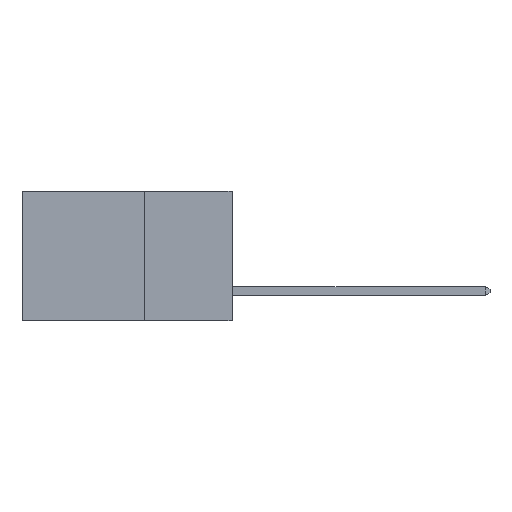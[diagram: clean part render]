
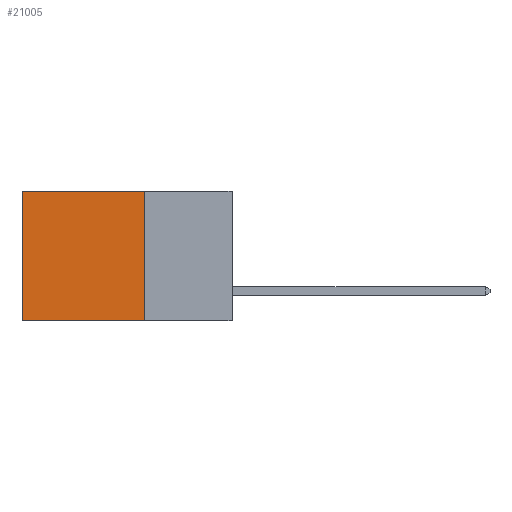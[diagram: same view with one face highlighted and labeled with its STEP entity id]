
A CAD part, left-side view. The second image highlights one B-rep face of the part: STEP entity #21005.
In plain terms, the highlighted planar face has unit normal (-1, 0, 0).
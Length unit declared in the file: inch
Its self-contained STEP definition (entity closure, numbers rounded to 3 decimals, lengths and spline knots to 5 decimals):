
#4359 = CARTESIAN_POINT ( 'NONE',  ( 0.2875, 0.25, 0. ) ) ;
#5199 = CARTESIAN_POINT ( 'NONE',  ( 0.2875, 0.25, 0. ) ) ;
#5298 = VERTEX_POINT ( 'NONE', #25255 ) ;
#5741 = DIRECTION ( 'NONE',  ( 0., 0., -1. ) ) ;
#5998 = ORIENTED_EDGE ( 'NONE', *, *, #12884, .T. ) ;
#7181 = AXIS2_PLACEMENT_3D ( 'NONE', #5199, #23310, #9797 ) ;
#7205 = DIRECTION ( 'NONE',  ( 0., 1., 0. ) ) ;
#8519 = EDGE_CURVE ( 'NONE', #5298, #20325, #26941, .T. ) ;
#8591 = CARTESIAN_POINT ( 'NONE',  ( 0.2875, 0.25, 0. ) ) ;
#9375 = EDGE_CURVE ( 'NONE', #25723, #20325, #21556, .T. ) ;
#9575 = VECTOR ( 'NONE', #5741, 39.37008 ) ;
#9644 = VECTOR ( 'NONE', #26665, 39.37008 ) ;
#9797 = DIRECTION ( 'NONE',  ( 0., 0., -1. ) ) ;
#10472 = VECTOR ( 'NONE', #22512, 39.37008 ) ;
#11093 = CARTESIAN_POINT ( 'NONE',  ( 0.2875, 0.6, 0. ) ) ;
#12884 = EDGE_CURVE ( 'NONE', #27003, #25723, #17109, .T. ) ;
#15580 = LINE ( 'NONE', #8591, #9644 ) ;
#15649 = CARTESIAN_POINT ( 'NONE',  ( 0.2875, 0.25, 0. ) ) ;
#17109 = LINE ( 'NONE', #4359, #10472 ) ;
#20325 = VERTEX_POINT ( 'NONE', #20544 ) ;
#20544 = CARTESIAN_POINT ( 'NONE',  ( 0.2875, 0.6, -0.37 ) ) ;
#20669 = CARTESIAN_POINT ( 'NONE',  ( 0.2875, 0.25, -0.37 ) ) ;
#20706 = ORIENTED_EDGE ( 'NONE', *, *, #9375, .T. ) ;
#20893 = VECTOR ( 'NONE', #7205, 39.37008 ) ;
#21005 = ADVANCED_FACE ( 'NONE', ( #21381 ), #21012, .F. ) ;
#21012 = PLANE ( 'NONE',  #7181 ) ;
#21381 = FACE_OUTER_BOUND ( 'NONE', #26900, .T. ) ;
#21556 = LINE ( 'NONE', #26003, #9575 ) ;
#21849 = ORIENTED_EDGE ( 'NONE', *, *, #24108, .F. ) ;
#22512 = DIRECTION ( 'NONE',  ( 0., 1., 0. ) ) ;
#23310 = DIRECTION ( 'NONE',  ( 1., 0., 0. ) ) ;
#24108 = EDGE_CURVE ( 'NONE', #27003, #5298, #15580, .T. ) ;
#24202 = ORIENTED_EDGE ( 'NONE', *, *, #8519, .F. ) ;
#25255 = CARTESIAN_POINT ( 'NONE',  ( 0.2875, 0.25, -0.37 ) ) ;
#25723 = VERTEX_POINT ( 'NONE', #11093 ) ;
#26003 = CARTESIAN_POINT ( 'NONE',  ( 0.2875, 0.6, 0. ) ) ;
#26665 = DIRECTION ( 'NONE',  ( 0., 0., -1. ) ) ;
#26900 = EDGE_LOOP ( 'NONE', ( #20706, #24202, #21849, #5998 ) ) ;
#26941 = LINE ( 'NONE', #20669, #20893 ) ;
#27003 = VERTEX_POINT ( 'NONE', #15649 ) ;
